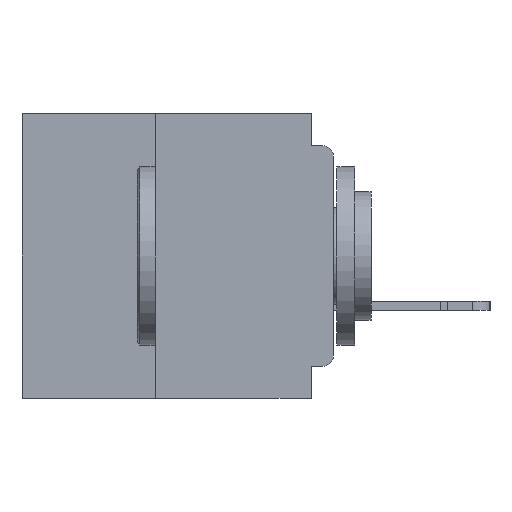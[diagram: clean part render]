
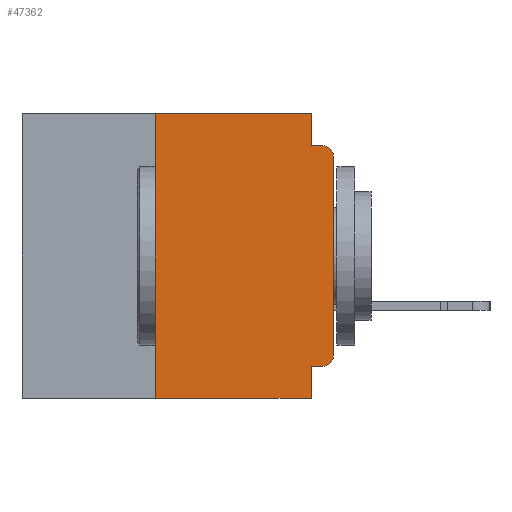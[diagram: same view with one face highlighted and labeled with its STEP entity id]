
A CAD part, left-side view. The second image highlights one B-rep face of the part: STEP entity #47362.
In plain terms, the highlighted planar face has unit normal (-1, 0, 0).
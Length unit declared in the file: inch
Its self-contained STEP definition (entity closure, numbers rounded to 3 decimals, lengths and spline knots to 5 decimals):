
#1317 = CARTESIAN_POINT ( 'NONE',  ( 0., 0.437, 0. ) ) ;
#2117 = DIRECTION ( 'NONE',  ( 0., 0., -1. ) ) ;
#2423 = LINE ( 'NONE', #50353, #29342 ) ;
#2746 = EDGE_CURVE ( 'NONE', #55826, #68001, #2423, .T. ) ;
#3476 = VECTOR ( 'NONE', #12000, 39.37008 ) ;
#3957 = EDGE_CURVE ( 'NONE', #41312, #19633, #33761, .T. ) ;
#5619 = VECTOR ( 'NONE', #2117, 39.37008 ) ;
#6910 = VECTOR ( 'NONE', #18134, 39.37008 ) ;
#8162 = CARTESIAN_POINT ( 'NONE',  ( 0., 0.437, 0. ) ) ;
#8620 = CARTESIAN_POINT ( 'NONE',  ( 0., 0.015, -0.34 ) ) ;
#8823 = ORIENTED_EDGE ( 'NONE', *, *, #9187, .F. ) ;
#8912 = CARTESIAN_POINT ( 'NONE',  ( 0., 0.031, -0.4 ) ) ;
#9187 = EDGE_CURVE ( 'NONE', #10663, #33269, #9344, .T. ) ;
#9344 = LINE ( 'NONE', #49373, #64462 ) ;
#10123 = ORIENTED_EDGE ( 'NONE', *, *, #30923, .T. ) ;
#10663 = VERTEX_POINT ( 'NONE', #49366 ) ;
#10726 = AXIS2_PLACEMENT_3D ( 'NONE', #8620, #46110, #14059 ) ;
#11135 = EDGE_CURVE ( 'NONE', #25343, #68001, #38378, .T. ) ;
#11402 = EDGE_CURVE ( 'NONE', #53976, #55826, #19948, .T. ) ;
#12000 = DIRECTION ( 'NONE',  ( 0., 0., 1. ) ) ;
#12375 = CARTESIAN_POINT ( 'NONE',  ( 0., 0.031, -0.045 ) ) ;
#12646 = CARTESIAN_POINT ( 'NONE',  ( 0., 0.25, -0.4 ) ) ;
#13605 = DIRECTION ( 'NONE',  ( 1., 0., 0. ) ) ;
#14059 = DIRECTION ( 'NONE',  ( 0., 0., -1. ) ) ;
#14406 = FACE_OUTER_BOUND ( 'NONE', #45801, .T. ) ;
#15119 = CARTESIAN_POINT ( 'NONE',  ( 0., 0.25, -0.4 ) ) ;
#17144 = AXIS2_PLACEMENT_3D ( 'NONE', #21466, #58798, #26840 ) ;
#18134 = DIRECTION ( 'NONE',  ( 0., 0., 1. ) ) ;
#19633 = VERTEX_POINT ( 'NONE', #65591 ) ;
#19675 = VECTOR ( 'NONE', #63979, 39.37008 ) ;
#19948 = LINE ( 'NONE', #28696, #5619 ) ;
#20105 = CARTESIAN_POINT ( 'NONE',  ( 0., 0., -0.34 ) ) ;
#20982 = CARTESIAN_POINT ( 'NONE',  ( 0., 0.015, -0.045 ) ) ;
#21311 = CARTESIAN_POINT ( 'NONE',  ( 0., 0.437, -0.4 ) ) ;
#21324 = VERTEX_POINT ( 'NONE', #20105 ) ;
#21333 = LINE ( 'NONE', #21311, #19675 ) ;
#21466 = CARTESIAN_POINT ( 'NONE',  ( 0., 0.015, -0.06 ) ) ;
#25343 = VERTEX_POINT ( 'NONE', #32107 ) ;
#26840 = DIRECTION ( 'NONE',  ( 0., 0., -1. ) ) ;
#27585 = VERTEX_POINT ( 'NONE', #42610 ) ;
#28696 = CARTESIAN_POINT ( 'NONE',  ( 0., 0.031, 0. ) ) ;
#28872 = CARTESIAN_POINT ( 'NONE',  ( 0., 0., 0. ) ) ;
#29342 = VECTOR ( 'NONE', #49887, 39.37008 ) ;
#29357 = EDGE_CURVE ( 'NONE', #41312, #33269, #21333, .T. ) ;
#30923 = EDGE_CURVE ( 'NONE', #21324, #25343, #62124, .T. ) ;
#32107 = CARTESIAN_POINT ( 'NONE',  ( 0., 0., -0.06 ) ) ;
#33269 = VERTEX_POINT ( 'NONE', #8912 ) ;
#33761 = LINE ( 'NONE', #12646, #3476 ) ;
#35351 = ORIENTED_EDGE ( 'NONE', *, *, #29357, .T. ) ;
#36225 = VECTOR ( 'NONE', #46873, 39.37008 ) ;
#38378 = CIRCLE ( 'NONE', #17144, 0.015 ) ;
#39891 = LINE ( 'NONE', #1317, #52400 ) ;
#40258 = ORIENTED_EDGE ( 'NONE', *, *, #63001, .F. ) ;
#41312 = VERTEX_POINT ( 'NONE', #15119 ) ;
#42610 = CARTESIAN_POINT ( 'NONE',  ( 0., 0.015, -0.355 ) ) ;
#44311 = DIRECTION ( 'NONE',  ( 0., -1., 0. ) ) ;
#45662 = PLANE ( 'NONE',  #66632 ) ;
#45801 = EDGE_LOOP ( 'NONE', ( #10123, #67864, #62733, #47617, #40258, #65850, #35351, #8823, #58223, #46881 ) ) ;
#46110 = DIRECTION ( 'NONE',  ( -1., 0., 0. ) ) ;
#46873 = DIRECTION ( 'NONE',  ( 0., 1., 0. ) ) ;
#46881 = ORIENTED_EDGE ( 'NONE', *, *, #57250, .T. ) ;
#47009 = EDGE_CURVE ( 'NONE', #27585, #10663, #52086, .T. ) ;
#47362 = ADVANCED_FACE ( 'NONE', ( #14406 ), #45662, .F. ) ;
#47617 = ORIENTED_EDGE ( 'NONE', *, *, #11402, .F. ) ;
#49366 = CARTESIAN_POINT ( 'NONE',  ( 0., 0.031, -0.355 ) ) ;
#49373 = CARTESIAN_POINT ( 'NONE',  ( 0., 0.031, -0.4 ) ) ;
#49887 = DIRECTION ( 'NONE',  ( 0., -1., 0. ) ) ;
#50353 = CARTESIAN_POINT ( 'NONE',  ( 0., 0., -0.045 ) ) ;
#50563 = CIRCLE ( 'NONE', #10726, 0.015 ) ;
#51016 = DIRECTION ( 'NONE',  ( 0., 0., -1. ) ) ;
#52086 = LINE ( 'NONE', #62657, #36225 ) ;
#52400 = VECTOR ( 'NONE', #44311, 39.37008 ) ;
#53976 = VERTEX_POINT ( 'NONE', #56429 ) ;
#55826 = VERTEX_POINT ( 'NONE', #12375 ) ;
#56429 = CARTESIAN_POINT ( 'NONE',  ( 0., 0.031, 0. ) ) ;
#57250 = EDGE_CURVE ( 'NONE', #27585, #21324, #50563, .T. ) ;
#58223 = ORIENTED_EDGE ( 'NONE', *, *, #47009, .F. ) ;
#58798 = DIRECTION ( 'NONE',  ( -1., 0., 0. ) ) ;
#62124 = LINE ( 'NONE', #28872, #6910 ) ;
#62657 = CARTESIAN_POINT ( 'NONE',  ( 0., 0., -0.355 ) ) ;
#62733 = ORIENTED_EDGE ( 'NONE', *, *, #2746, .F. ) ;
#63001 = EDGE_CURVE ( 'NONE', #19633, #53976, #39891, .T. ) ;
#63979 = DIRECTION ( 'NONE',  ( 0., -1., 0. ) ) ;
#64462 = VECTOR ( 'NONE', #65366, 39.37008 ) ;
#65366 = DIRECTION ( 'NONE',  ( 0., 0., -1. ) ) ;
#65591 = CARTESIAN_POINT ( 'NONE',  ( 0., 0.25, 0. ) ) ;
#65850 = ORIENTED_EDGE ( 'NONE', *, *, #3957, .F. ) ;
#66632 = AXIS2_PLACEMENT_3D ( 'NONE', #8162, #13605, #51016 ) ;
#67864 = ORIENTED_EDGE ( 'NONE', *, *, #11135, .T. ) ;
#68001 = VERTEX_POINT ( 'NONE', #20982 ) ;
